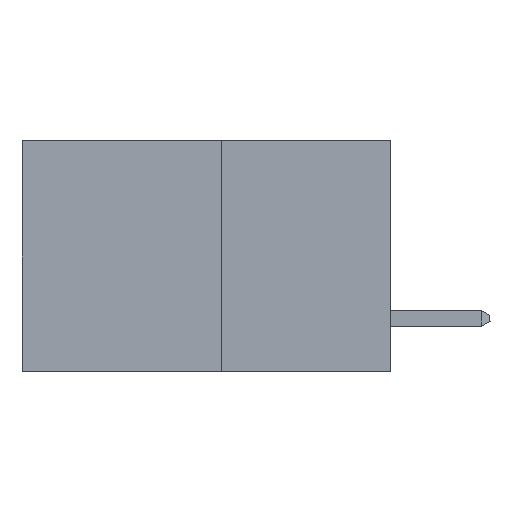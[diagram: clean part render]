
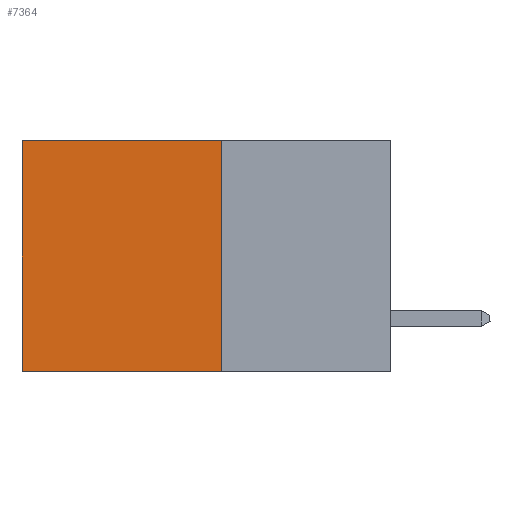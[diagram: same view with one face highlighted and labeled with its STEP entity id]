
A CAD part, left-side view. The second image highlights one B-rep face of the part: STEP entity #7364.
In plain terms, the highlighted planar face has unit normal (-1, 0, 0).
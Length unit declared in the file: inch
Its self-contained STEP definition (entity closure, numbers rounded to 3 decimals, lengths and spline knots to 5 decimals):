
#443 = DIRECTION ( 'NONE',  ( 0., 0., -1. ) ) ;
#1191 = FACE_OUTER_BOUND ( 'NONE', #2994, .T. ) ;
#1298 = CARTESIAN_POINT ( 'NONE',  ( 0.277, 0.59, -0.37 ) ) ;
#1697 = DIRECTION ( 'NONE',  ( 0., 1., 0. ) ) ;
#1701 = EDGE_CURVE ( 'NONE', #6864, #8918, #7128, .T. ) ;
#1871 = ORIENTED_EDGE ( 'NONE', *, *, #2329, .T. ) ;
#2320 = CARTESIAN_POINT ( 'NONE',  ( 0.277, 0.27, -0.37 ) ) ;
#2329 = EDGE_CURVE ( 'NONE', #11105, #5157, #6605, .T. ) ;
#2951 = CARTESIAN_POINT ( 'NONE',  ( 0.277, 0.59, -0.37 ) ) ;
#2994 = EDGE_LOOP ( 'NONE', ( #13654, #10831, #13271, #1871 ) ) ;
#3452 = CARTESIAN_POINT ( 'NONE',  ( 0.277, 0.27, -0.37 ) ) ;
#3667 = CARTESIAN_POINT ( 'NONE',  ( 0.277, 0.27, -0.37 ) ) ;
#4731 = CARTESIAN_POINT ( 'NONE',  ( 0.277, 0.27, -0.37 ) ) ;
#5157 = VERTEX_POINT ( 'NONE', #14524 ) ;
#5687 = AXIS2_PLACEMENT_3D ( 'NONE', #4731, #8733, #443 ) ;
#6605 = LINE ( 'NONE', #13676, #13684 ) ;
#6797 = EDGE_CURVE ( 'NONE', #11105, #6864, #8292, .T. ) ;
#6864 = VERTEX_POINT ( 'NONE', #2320 ) ;
#7128 = LINE ( 'NONE', #3452, #9874 ) ;
#7364 = ADVANCED_FACE ( 'NONE', ( #1191 ), #7414, .F. ) ;
#7414 = PLANE ( 'NONE',  #5687 ) ;
#7984 = LINE ( 'NONE', #1298, #11532 ) ;
#8292 = LINE ( 'NONE', #3667, #13106 ) ;
#8733 = DIRECTION ( 'NONE',  ( 1., 0., 0. ) ) ;
#8918 = VERTEX_POINT ( 'NONE', #2951 ) ;
#9874 = VECTOR ( 'NONE', #1697, 39.37008 ) ;
#10365 = DIRECTION ( 'NONE',  ( 0., 0., -1. ) ) ;
#10831 = ORIENTED_EDGE ( 'NONE', *, *, #1701, .F. ) ;
#11105 = VERTEX_POINT ( 'NONE', #12786 ) ;
#11520 = EDGE_CURVE ( 'NONE', #5157, #8918, #7984, .T. ) ;
#11532 = VECTOR ( 'NONE', #13524, 39.37008 ) ;
#12786 = CARTESIAN_POINT ( 'NONE',  ( 0.277, 0.27, 0. ) ) ;
#13106 = VECTOR ( 'NONE', #10365, 39.37008 ) ;
#13271 = ORIENTED_EDGE ( 'NONE', *, *, #6797, .F. ) ;
#13524 = DIRECTION ( 'NONE',  ( 0., 0., -1. ) ) ;
#13554 = DIRECTION ( 'NONE',  ( 0., 1., 0. ) ) ;
#13654 = ORIENTED_EDGE ( 'NONE', *, *, #11520, .T. ) ;
#13676 = CARTESIAN_POINT ( 'NONE',  ( 0.277, 0.27, 0. ) ) ;
#13684 = VECTOR ( 'NONE', #13554, 39.37008 ) ;
#14524 = CARTESIAN_POINT ( 'NONE',  ( 0.277, 0.59, 0. ) ) ;
